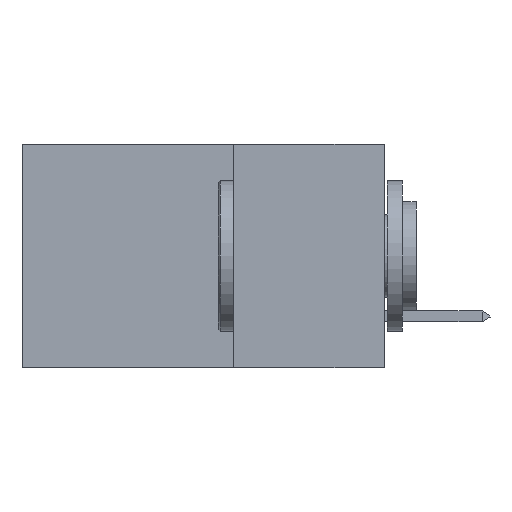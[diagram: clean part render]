
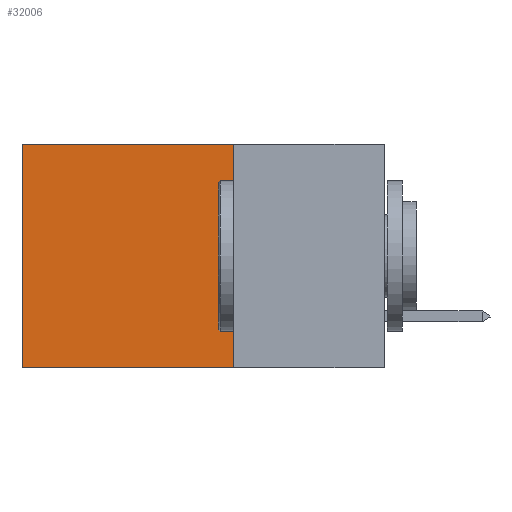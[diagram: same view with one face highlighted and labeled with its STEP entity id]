
A CAD part, left-side view. The second image highlights one B-rep face of the part: STEP entity #32006.
In plain terms, the highlighted planar face has unit normal (-1, 0, 0).
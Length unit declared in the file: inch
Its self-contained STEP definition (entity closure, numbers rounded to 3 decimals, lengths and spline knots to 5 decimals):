
#1797 = CARTESIAN_POINT ( 'NONE',  ( 0.2875, 0.25, -0.37 ) ) ;
#2168 = CARTESIAN_POINT ( 'NONE',  ( 0.2875, 0.25, -0.37 ) ) ;
#2287 = LINE ( 'NONE', #3746, #4497 ) ;
#3746 = CARTESIAN_POINT ( 'NONE',  ( 0.2875, 0.6, 0. ) ) ;
#4497 = VECTOR ( 'NONE', #18322, 39.37008 ) ;
#4567 = CARTESIAN_POINT ( 'NONE',  ( 0.2875, 0.25, 0. ) ) ;
#4885 = VERTEX_POINT ( 'NONE', #14612 ) ;
#5357 = LINE ( 'NONE', #4567, #33334 ) ;
#6231 = EDGE_CURVE ( 'NONE', #19271, #39943, #2287, .T. ) ;
#6907 = EDGE_LOOP ( 'NONE', ( #24531, #9063, #14513, #31710 ) ) ;
#9063 = ORIENTED_EDGE ( 'NONE', *, *, #46342, .F. ) ;
#10584 = AXIS2_PLACEMENT_3D ( 'NONE', #27627, #45387, #23651 ) ;
#10961 = CARTESIAN_POINT ( 'NONE',  ( 0.2875, 0.6, -0.37 ) ) ;
#11862 = CARTESIAN_POINT ( 'NONE',  ( 0.2875, 0.6, 0. ) ) ;
#14513 = ORIENTED_EDGE ( 'NONE', *, *, #32408, .F. ) ;
#14612 = CARTESIAN_POINT ( 'NONE',  ( 0.2875, 0.25, 0. ) ) ;
#18322 = DIRECTION ( 'NONE',  ( 0., 0., -1. ) ) ;
#19271 = VERTEX_POINT ( 'NONE', #11862 ) ;
#19297 = DIRECTION ( 'NONE',  ( 0., 0., -1. ) ) ;
#20419 = DIRECTION ( 'NONE',  ( 0., 1., 0. ) ) ;
#23651 = DIRECTION ( 'NONE',  ( 0., 0., -1. ) ) ;
#23747 = CARTESIAN_POINT ( 'NONE',  ( 0.2875, 0.25, 0. ) ) ;
#24531 = ORIENTED_EDGE ( 'NONE', *, *, #6231, .T. ) ;
#27385 = DIRECTION ( 'NONE',  ( 0., 1., 0. ) ) ;
#27627 = CARTESIAN_POINT ( 'NONE',  ( 0.2875, 0.25, 0. ) ) ;
#30246 = EDGE_CURVE ( 'NONE', #4885, #19271, #44907, .T. ) ;
#30729 = VECTOR ( 'NONE', #20419, 39.37008 ) ;
#31710 = ORIENTED_EDGE ( 'NONE', *, *, #30246, .T. ) ;
#32006 = ADVANCED_FACE ( 'NONE', ( #44728 ), #34768, .F. ) ;
#32408 = EDGE_CURVE ( 'NONE', #4885, #46998, #5357, .T. ) ;
#33334 = VECTOR ( 'NONE', #19297, 39.37008 ) ;
#34768 = PLANE ( 'NONE',  #10584 ) ;
#36679 = LINE ( 'NONE', #2168, #44601 ) ;
#39943 = VERTEX_POINT ( 'NONE', #10961 ) ;
#44601 = VECTOR ( 'NONE', #27385, 39.37008 ) ;
#44728 = FACE_OUTER_BOUND ( 'NONE', #6907, .T. ) ;
#44907 = LINE ( 'NONE', #23747, #30729 ) ;
#45387 = DIRECTION ( 'NONE',  ( 1., 0., 0. ) ) ;
#46342 = EDGE_CURVE ( 'NONE', #46998, #39943, #36679, .T. ) ;
#46998 = VERTEX_POINT ( 'NONE', #1797 ) ;
